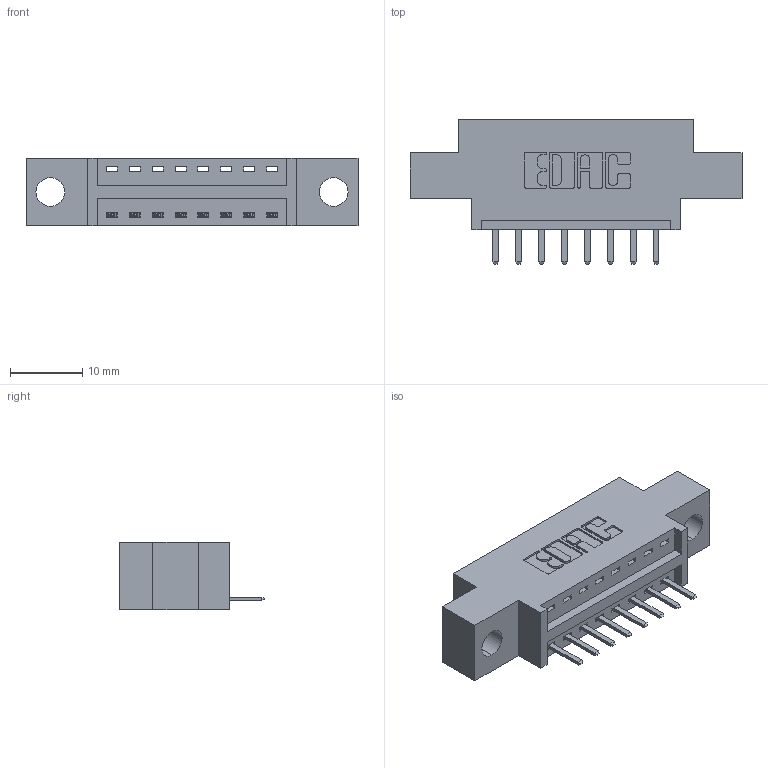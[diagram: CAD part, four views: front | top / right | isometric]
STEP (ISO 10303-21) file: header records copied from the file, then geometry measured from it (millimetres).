
FILE_DESCRIPTION (( 'STEP AP203' ), '1' );
FILE_NAME ('346-008-520-604.STEP', '2022-05-04T20:45:20', ( '' ), ( '' ), 'SwSTEP 2.0', 'SolidWorks 2020', '' );
FILE_SCHEMA (( 'CONFIG_CONTROL_DESIGN' ));
Length unit declared in the file: inch
Products named in the file (3): 346-008-520-604; 346 Part_0.170 Offset - 0.156 Dia-TH; 345-292-001_345-293-120
Assembly tree (9 placements, depth 2):
  346-008-520-604
    346 Part_0.170 Offset - 0.156 Dia-TH
    345-292-001_345-293-120  x8
Bounding box: 45.97 x 20.02 x 9.4 mm (x, y, z)
Volume: 3882.9 mm3; surface area: 4407 mm2
Topology: 9 solids, 9 shells, 636 faces, 1849 edges, 1210 vertices
Faces by surface type: plane 430, cylinder 206
Entity records: 10207 total; most frequent: CARTESIAN_POINT 1782, ORIENTED_EDGE 1710, DIRECTION 1599, EDGE_CURVE 855, VECTOR 687, LINE 687, VERTEX_POINT 566, AXIS2_PLACEMENT_3D 456
